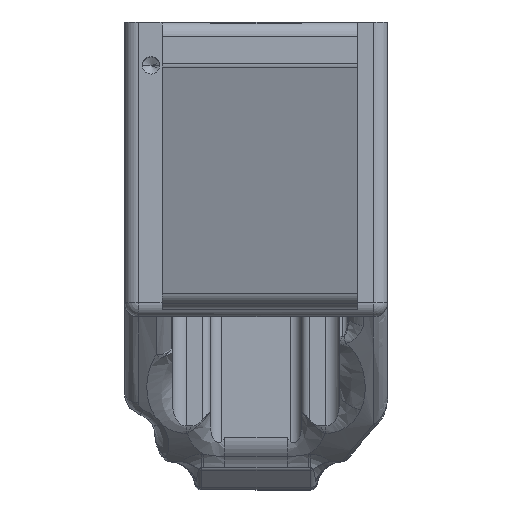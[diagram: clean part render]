
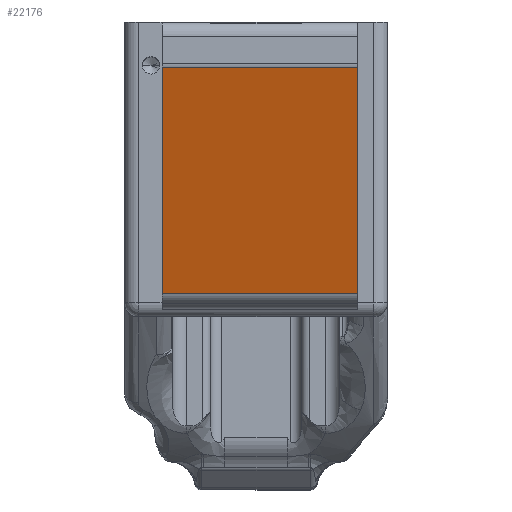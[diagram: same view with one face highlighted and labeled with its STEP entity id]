
A CAD part, top view. The second image highlights one B-rep face of the part: STEP entity #22176.
In plain terms, the highlighted planar face has unit normal (0, -0.287, 0.958).
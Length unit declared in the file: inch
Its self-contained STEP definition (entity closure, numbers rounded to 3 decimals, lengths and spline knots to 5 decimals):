
#758 = DIRECTION ( 'NONE',  ( -1., 0., 0. ) ) ;
#1266 = CARTESIAN_POINT ( 'NONE',  ( 0.20897, -0.17969, 3.20707 ) ) ;
#1303 = DIRECTION ( 'NONE',  ( 0., 0.958, 0.287 ) ) ;
#2711 = LINE ( 'NONE', #9622, #10119 ) ;
#3043 = EDGE_CURVE ( 'NONE', #7143, #15166, #6365, .T. ) ;
#3170 = VERTEX_POINT ( 'NONE', #5402 ) ;
#3757 = EDGE_LOOP ( 'NONE', ( #8735, #13765, #20752, #23476 ) ) ;
#5402 = CARTESIAN_POINT ( 'NONE',  ( 1.29347, 1.07844, 3.58419 ) ) ;
#6365 = LINE ( 'NONE', #9033, #11964 ) ;
#6878 = DIRECTION ( 'NONE',  ( -1., 0., 0. ) ) ;
#7143 = VERTEX_POINT ( 'NONE', #8328 ) ;
#8310 = CARTESIAN_POINT ( 'NONE',  ( 2.03801, -0.17969, 3.20707 ) ) ;
#8328 = CARTESIAN_POINT ( 'NONE',  ( 0.20897, 1.07844, 3.58419 ) ) ;
#8735 = ORIENTED_EDGE ( 'NONE', *, *, #24493, .F. ) ;
#9033 = CARTESIAN_POINT ( 'NONE',  ( 0.20897, -0.89688, 2.99209 ) ) ;
#9622 = CARTESIAN_POINT ( 'NONE',  ( 1.29347, 1.07844, 3.58419 ) ) ;
#10119 = VECTOR ( 'NONE', #13428, 39.37008 ) ;
#10591 = CARTESIAN_POINT ( 'NONE',  ( 0.20897, 1.07844, 3.58419 ) ) ;
#10748 = PLANE ( 'NONE',  #19862 ) ;
#10749 = VECTOR ( 'NONE', #6878, 39.37008 ) ;
#11636 = VERTEX_POINT ( 'NONE', #17940 ) ;
#11964 = VECTOR ( 'NONE', #24241, 39.37008 ) ;
#12647 = DIRECTION ( 'NONE',  ( 0., 0.287, -0.958 ) ) ;
#13100 = VECTOR ( 'NONE', #758, 39.37008 ) ;
#13428 = DIRECTION ( 'NONE',  ( 0., -0.958, -0.287 ) ) ;
#13765 = ORIENTED_EDGE ( 'NONE', *, *, #14591, .F. ) ;
#14591 = EDGE_CURVE ( 'NONE', #3170, #11636, #2711, .T. ) ;
#15166 = VERTEX_POINT ( 'NONE', #1266 ) ;
#16255 = FACE_OUTER_BOUND ( 'NONE', #3757, .T. ) ;
#17940 = CARTESIAN_POINT ( 'NONE',  ( 1.29347, -0.17969, 3.20707 ) ) ;
#17997 = EDGE_CURVE ( 'NONE', #3170, #7143, #22025, .T. ) ;
#18145 = LINE ( 'NONE', #8310, #13100 ) ;
#18208 = CARTESIAN_POINT ( 'NONE',  ( 2.03801, -0.89688, 2.99209 ) ) ;
#19862 = AXIS2_PLACEMENT_3D ( 'NONE', #18208, #12647, #1303 ) ;
#20752 = ORIENTED_EDGE ( 'NONE', *, *, #17997, .T. ) ;
#22025 = LINE ( 'NONE', #10591, #10749 ) ;
#22176 = ADVANCED_FACE ( 'NONE', ( #16255 ), #10748, .F. ) ;
#23476 = ORIENTED_EDGE ( 'NONE', *, *, #3043, .T. ) ;
#24241 = DIRECTION ( 'NONE',  ( 0., -0.958, -0.287 ) ) ;
#24493 = EDGE_CURVE ( 'NONE', #11636, #15166, #18145, .T. ) ;
